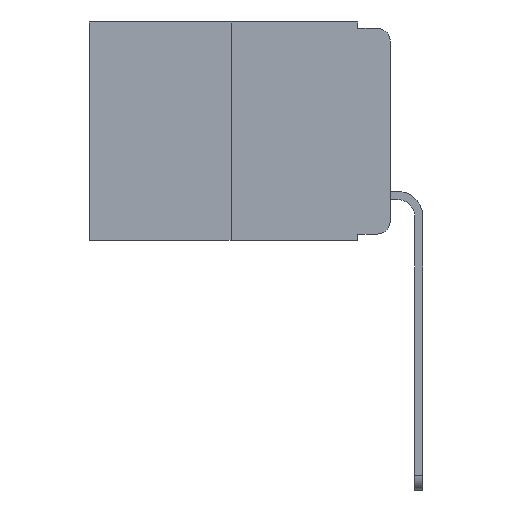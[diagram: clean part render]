
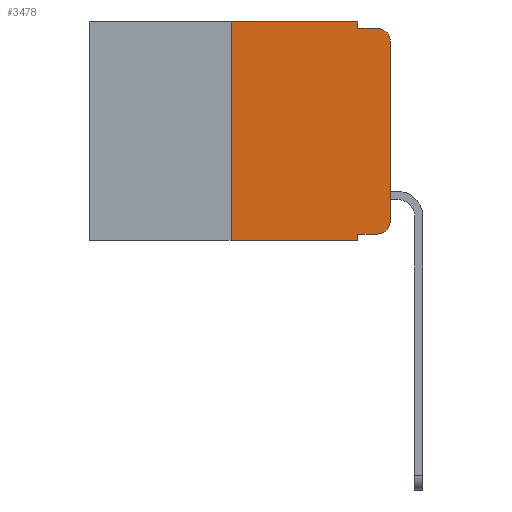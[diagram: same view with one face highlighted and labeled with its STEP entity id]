
A CAD part, left-side view. The second image highlights one B-rep face of the part: STEP entity #3478.
In plain terms, the highlighted planar face has unit normal (-1, 0, 0).
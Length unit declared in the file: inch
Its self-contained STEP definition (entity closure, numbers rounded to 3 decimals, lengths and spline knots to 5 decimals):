
#218 = CARTESIAN_POINT ( 'NONE',  ( 0., 0.051, -0.343 ) ) ;
#425 = VERTEX_POINT ( 'NONE', #11572 ) ;
#474 = VERTEX_POINT ( 'NONE', #8894 ) ;
#642 = VERTEX_POINT ( 'NONE', #9441 ) ;
#791 = ORIENTED_EDGE ( 'NONE', *, *, #5649, .F. ) ;
#856 = CARTESIAN_POINT ( 'NONE',  ( 0., 0.051, 0. ) ) ;
#1007 = CARTESIAN_POINT ( 'NONE',  ( 0., 0.051, 0. ) ) ;
#1081 = ORIENTED_EDGE ( 'NONE', *, *, #8320, .F. ) ;
#1404 = ORIENTED_EDGE ( 'NONE', *, *, #8371, .F. ) ;
#1407 = VECTOR ( 'NONE', #10766, 39.37008 ) ;
#1486 = ORIENTED_EDGE ( 'NONE', *, *, #11295, .T. ) ;
#2005 = AXIS2_PLACEMENT_3D ( 'NONE', #5168, #6993, #3444 ) ;
#2014 = EDGE_CURVE ( 'NONE', #3991, #2782, #7692, .T. ) ;
#2423 = CARTESIAN_POINT ( 'NONE',  ( 0., 0.473, 0. ) ) ;
#2451 = VECTOR ( 'NONE', #9792, 39.37008 ) ;
#2595 = CARTESIAN_POINT ( 'NONE',  ( 0., 0.25, 0. ) ) ;
#2782 = VERTEX_POINT ( 'NONE', #5583 ) ;
#3120 = ORIENTED_EDGE ( 'NONE', *, *, #2014, .T. ) ;
#3189 = CARTESIAN_POINT ( 'NONE',  ( 0., 0., -0.313 ) ) ;
#3190 = VECTOR ( 'NONE', #9610, 39.37008 ) ;
#3257 = VERTEX_POINT ( 'NONE', #3610 ) ;
#3356 = VERTEX_POINT ( 'NONE', #218 ) ;
#3444 = DIRECTION ( 'NONE',  ( 0., 0., -1. ) ) ;
#3478 = ADVANCED_FACE ( 'NONE', ( #7943 ), #4107, .F. ) ;
#3532 = LINE ( 'NONE', #2595, #5489 ) ;
#3535 = CARTESIAN_POINT ( 'NONE',  ( 0., 0.051, 0. ) ) ;
#3556 = DIRECTION ( 'NONE',  ( 0., -1., 0. ) ) ;
#3610 = CARTESIAN_POINT ( 'NONE',  ( 0., 0.02, -0.333 ) ) ;
#3636 = LINE ( 'NONE', #6867, #4034 ) ;
#3983 = CARTESIAN_POINT ( 'NONE',  ( 0., 0., 0. ) ) ;
#3991 = VERTEX_POINT ( 'NONE', #8377 ) ;
#4034 = VECTOR ( 'NONE', #10309, 39.37008 ) ;
#4040 = CARTESIAN_POINT ( 'NONE',  ( 0., 0.473, 0. ) ) ;
#4107 = PLANE ( 'NONE',  #9899 ) ;
#4110 = LINE ( 'NONE', #8956, #10837 ) ;
#4134 = LINE ( 'NONE', #856, #2451 ) ;
#4176 = VECTOR ( 'NONE', #3556, 39.37008 ) ;
#4517 = CARTESIAN_POINT ( 'NONE',  ( 0., 0.051, -0.333 ) ) ;
#4584 = EDGE_CURVE ( 'NONE', #4758, #3991, #8746, .T. ) ;
#4753 = EDGE_CURVE ( 'NONE', #8363, #2782, #3636, .T. ) ;
#4758 = VERTEX_POINT ( 'NONE', #3189 ) ;
#4842 = DIRECTION ( 'NONE',  ( 0., 0., 1. ) ) ;
#4952 = ORIENTED_EDGE ( 'NONE', *, *, #11137, .F. ) ;
#5168 = CARTESIAN_POINT ( 'NONE',  ( 0., 0.02, -0.03 ) ) ;
#5257 = VECTOR ( 'NONE', #4842, 39.37008 ) ;
#5336 = DIRECTION ( 'NONE',  ( 0., -1., 0. ) ) ;
#5364 = DIRECTION ( 'NONE',  ( -1., 0., 0. ) ) ;
#5405 = CARTESIAN_POINT ( 'NONE',  ( 0., 0.051, -0.01 ) ) ;
#5489 = VECTOR ( 'NONE', #9733, 39.37008 ) ;
#5583 = CARTESIAN_POINT ( 'NONE',  ( 0., 0.02, -0.01 ) ) ;
#5649 = EDGE_CURVE ( 'NONE', #642, #3356, #4134, .T. ) ;
#6331 = EDGE_CURVE ( 'NONE', #474, #3356, #4110, .T. ) ;
#6485 = ORIENTED_EDGE ( 'NONE', *, *, #6331, .T. ) ;
#6509 = AXIS2_PLACEMENT_3D ( 'NONE', #9730, #5364, #7114 ) ;
#6763 = CIRCLE ( 'NONE', #6509, 0.02 ) ;
#6867 = CARTESIAN_POINT ( 'NONE',  ( 0., 0.051, -0.01 ) ) ;
#6993 = DIRECTION ( 'NONE',  ( -1., 0., 0. ) ) ;
#7114 = DIRECTION ( 'NONE',  ( 0., 0., -1. ) ) ;
#7321 = ORIENTED_EDGE ( 'NONE', *, *, #7858, .T. ) ;
#7535 = ORIENTED_EDGE ( 'NONE', *, *, #4584, .T. ) ;
#7692 = CIRCLE ( 'NONE', #2005, 0.02 ) ;
#7858 = EDGE_CURVE ( 'NONE', #3257, #4758, #6763, .T. ) ;
#7943 = FACE_OUTER_BOUND ( 'NONE', #11257, .T. ) ;
#8282 = VERTEX_POINT ( 'NONE', #3535 ) ;
#8320 = EDGE_CURVE ( 'NONE', #474, #425, #3532, .T. ) ;
#8363 = VERTEX_POINT ( 'NONE', #5405 ) ;
#8371 = EDGE_CURVE ( 'NONE', #8282, #8363, #10797, .T. ) ;
#8377 = CARTESIAN_POINT ( 'NONE',  ( 0., 0., -0.03 ) ) ;
#8541 = DIRECTION ( 'NONE',  ( 0., 0., -1. ) ) ;
#8646 = ORIENTED_EDGE ( 'NONE', *, *, #4753, .F. ) ;
#8746 = LINE ( 'NONE', #3983, #5257 ) ;
#8894 = CARTESIAN_POINT ( 'NONE',  ( 0., 0.25, -0.343 ) ) ;
#8956 = CARTESIAN_POINT ( 'NONE',  ( 0., 0.473, -0.343 ) ) ;
#9441 = CARTESIAN_POINT ( 'NONE',  ( 0., 0.051, -0.333 ) ) ;
#9610 = DIRECTION ( 'NONE',  ( 0., -1., 0. ) ) ;
#9730 = CARTESIAN_POINT ( 'NONE',  ( 0., 0.02, -0.313 ) ) ;
#9733 = DIRECTION ( 'NONE',  ( 0., 0., 1. ) ) ;
#9792 = DIRECTION ( 'NONE',  ( 0., 0., -1. ) ) ;
#9899 = AXIS2_PLACEMENT_3D ( 'NONE', #4040, #10335, #8541 ) ;
#10309 = DIRECTION ( 'NONE',  ( 0., -1., 0. ) ) ;
#10335 = DIRECTION ( 'NONE',  ( 1., 0., 0. ) ) ;
#10766 = DIRECTION ( 'NONE',  ( 0., 0., -1. ) ) ;
#10797 = LINE ( 'NONE', #1007, #1407 ) ;
#10837 = VECTOR ( 'NONE', #5336, 39.37008 ) ;
#11137 = EDGE_CURVE ( 'NONE', #425, #8282, #11304, .T. ) ;
#11257 = EDGE_LOOP ( 'NONE', ( #7535, #3120, #8646, #1404, #4952, #1081, #6485, #791, #1486, #7321 ) ) ;
#11295 = EDGE_CURVE ( 'NONE', #642, #3257, #11460, .T. ) ;
#11304 = LINE ( 'NONE', #2423, #3190 ) ;
#11460 = LINE ( 'NONE', #4517, #4176 ) ;
#11572 = CARTESIAN_POINT ( 'NONE',  ( 0., 0.25, 0. ) ) ;
